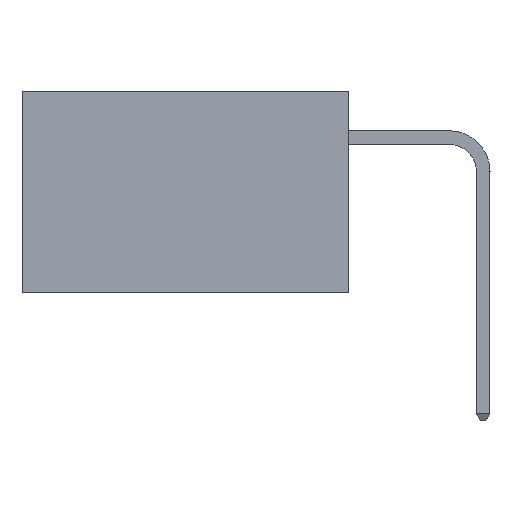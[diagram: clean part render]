
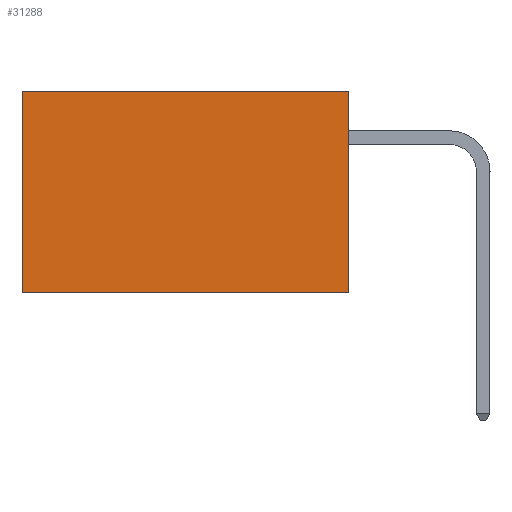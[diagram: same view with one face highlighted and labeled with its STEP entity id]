
A CAD part, left-side view. The second image highlights one B-rep face of the part: STEP entity #31288.
In plain terms, the highlighted planar face has unit normal (-1, 0, 0).
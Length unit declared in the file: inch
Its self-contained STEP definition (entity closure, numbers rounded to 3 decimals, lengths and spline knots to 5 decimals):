
#886 = EDGE_CURVE ( 'NONE', #2604, #17029, #4128, .T. ) ;
#1004 = DIRECTION ( 'NONE',  ( 0., 1., 0. ) ) ;
#1236 = FACE_OUTER_BOUND ( 'NONE', #4620, .T. ) ;
#2202 = EDGE_CURVE ( 'NONE', #17029, #20973, #14625, .T. ) ;
#2604 = VERTEX_POINT ( 'NONE', #26516 ) ;
#2911 = DIRECTION ( 'NONE',  ( 0., 1., 0. ) ) ;
#3553 = PLANE ( 'NONE',  #8988 ) ;
#3613 = ORIENTED_EDGE ( 'NONE', *, *, #8779, .F. ) ;
#4128 = LINE ( 'NONE', #19241, #31122 ) ;
#4620 = EDGE_LOOP ( 'NONE', ( #21828, #13509, #3613, #35012 ) ) ;
#4711 = LINE ( 'NONE', #18645, #33412 ) ;
#5253 = LINE ( 'NONE', #15070, #33954 ) ;
#6192 = CARTESIAN_POINT ( 'NONE',  ( 0.2875, 0., -0.37 ) ) ;
#6292 = CARTESIAN_POINT ( 'NONE',  ( 0.2875, 0.6, 0. ) ) ;
#8779 = EDGE_CURVE ( 'NONE', #2604, #34558, #4711, .T. ) ;
#8988 = AXIS2_PLACEMENT_3D ( 'NONE', #17581, #34183, #17704 ) ;
#10286 = DIRECTION ( 'NONE',  ( 0., 0., -1. ) ) ;
#13509 = ORIENTED_EDGE ( 'NONE', *, *, #24629, .F. ) ;
#14625 = LINE ( 'NONE', #6292, #21145 ) ;
#15070 = CARTESIAN_POINT ( 'NONE',  ( 0.2875, 0., -0.37 ) ) ;
#17029 = VERTEX_POINT ( 'NONE', #22133 ) ;
#17581 = CARTESIAN_POINT ( 'NONE',  ( 0.2875, 0., 0. ) ) ;
#17704 = DIRECTION ( 'NONE',  ( 0., 0., -1. ) ) ;
#18645 = CARTESIAN_POINT ( 'NONE',  ( 0.2875, 0., 0. ) ) ;
#19241 = CARTESIAN_POINT ( 'NONE',  ( 0.2875, 0., 0. ) ) ;
#20973 = VERTEX_POINT ( 'NONE', #25693 ) ;
#21145 = VECTOR ( 'NONE', #31098, 39.37008 ) ;
#21828 = ORIENTED_EDGE ( 'NONE', *, *, #2202, .T. ) ;
#22133 = CARTESIAN_POINT ( 'NONE',  ( 0.2875, 0.6, 0. ) ) ;
#24629 = EDGE_CURVE ( 'NONE', #34558, #20973, #5253, .T. ) ;
#25693 = CARTESIAN_POINT ( 'NONE',  ( 0.2875, 0.6, -0.37 ) ) ;
#26516 = CARTESIAN_POINT ( 'NONE',  ( 0.2875, 0., 0. ) ) ;
#31098 = DIRECTION ( 'NONE',  ( 0., 0., -1. ) ) ;
#31122 = VECTOR ( 'NONE', #2911, 39.37008 ) ;
#31288 = ADVANCED_FACE ( 'NONE', ( #1236 ), #3553, .F. ) ;
#33412 = VECTOR ( 'NONE', #10286, 39.37008 ) ;
#33954 = VECTOR ( 'NONE', #1004, 39.37008 ) ;
#34183 = DIRECTION ( 'NONE',  ( 1., 0., 0. ) ) ;
#34558 = VERTEX_POINT ( 'NONE', #6192 ) ;
#35012 = ORIENTED_EDGE ( 'NONE', *, *, #886, .T. ) ;
